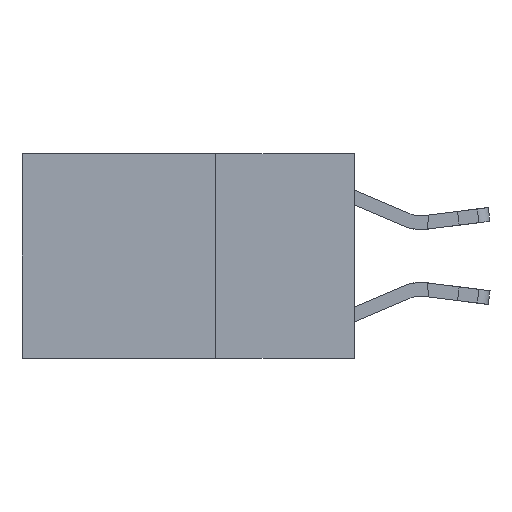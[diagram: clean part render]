
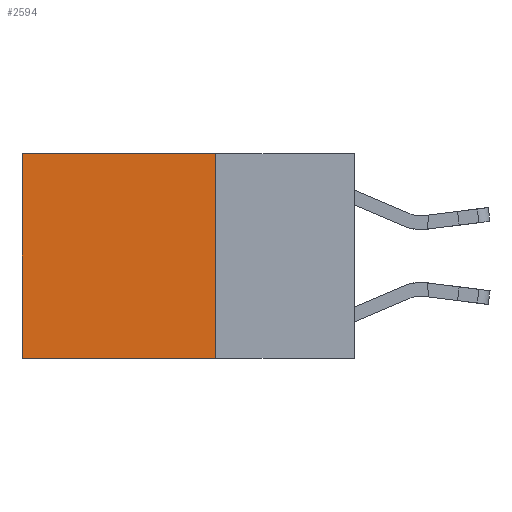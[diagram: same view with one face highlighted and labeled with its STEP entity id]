
A CAD part, left-side view. The second image highlights one B-rep face of the part: STEP entity #2594.
In plain terms, the highlighted planar face has unit normal (-1, 0, 0).
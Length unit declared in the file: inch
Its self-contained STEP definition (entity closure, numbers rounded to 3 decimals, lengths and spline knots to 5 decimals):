
#335 = ORIENTED_EDGE ( 'NONE', *, *, #14577, .F. ) ;
#1038 = FACE_OUTER_BOUND ( 'NONE', #13668, .T. ) ;
#1666 = PLANE ( 'NONE',  #3285 ) ;
#1735 = CARTESIAN_POINT ( 'NONE',  ( 0.2625, 0.25, 0. ) ) ;
#1909 = CARTESIAN_POINT ( 'NONE',  ( 0.2625, 0.6, 0. ) ) ;
#2092 = VERTEX_POINT ( 'NONE', #3716 ) ;
#2224 = EDGE_CURVE ( 'NONE', #2092, #17939, #18681, .T. ) ;
#2594 = ADVANCED_FACE ( 'NONE', ( #1038 ), #1666, .F. ) ;
#2650 = LINE ( 'NONE', #3391, #6215 ) ;
#3251 = DIRECTION ( 'NONE',  ( 0., 0., -1. ) ) ;
#3285 = AXIS2_PLACEMENT_3D ( 'NONE', #1735, #12367, #3251 ) ;
#3361 = CARTESIAN_POINT ( 'NONE',  ( 0.2625, 0.25, 0. ) ) ;
#3391 = CARTESIAN_POINT ( 'NONE',  ( 0.2625, 0.25, 0. ) ) ;
#3416 = DIRECTION ( 'NONE',  ( 0., 0., -1. ) ) ;
#3716 = CARTESIAN_POINT ( 'NONE',  ( 0.2625, 0.25, -0.37 ) ) ;
#4648 = ORIENTED_EDGE ( 'NONE', *, *, #13166, .T. ) ;
#6148 = LINE ( 'NONE', #1909, #14195 ) ;
#6215 = VECTOR ( 'NONE', #15488, 39.37008 ) ;
#7209 = CARTESIAN_POINT ( 'NONE',  ( 0.2625, 0.6, 0. ) ) ;
#7550 = DIRECTION ( 'NONE',  ( 0., 1., 0. ) ) ;
#7702 = VECTOR ( 'NONE', #17535, 39.37008 ) ;
#7861 = VERTEX_POINT ( 'NONE', #7209 ) ;
#7956 = CARTESIAN_POINT ( 'NONE',  ( 0.2625, 0.6, -0.37 ) ) ;
#9544 = EDGE_CURVE ( 'NONE', #7861, #17939, #6148, .T. ) ;
#10501 = ORIENTED_EDGE ( 'NONE', *, *, #9544, .T. ) ;
#11110 = ORIENTED_EDGE ( 'NONE', *, *, #2224, .F. ) ;
#12367 = DIRECTION ( 'NONE',  ( 1., 0., 0. ) ) ;
#12652 = VERTEX_POINT ( 'NONE', #3361 ) ;
#13166 = EDGE_CURVE ( 'NONE', #12652, #7861, #15707, .T. ) ;
#13668 = EDGE_LOOP ( 'NONE', ( #10501, #11110, #335, #4648 ) ) ;
#14195 = VECTOR ( 'NONE', #3416, 39.37008 ) ;
#14577 = EDGE_CURVE ( 'NONE', #12652, #2092, #2650, .T. ) ;
#15488 = DIRECTION ( 'NONE',  ( 0., 0., -1. ) ) ;
#15515 = CARTESIAN_POINT ( 'NONE',  ( 0.2625, 0.25, 0. ) ) ;
#15707 = LINE ( 'NONE', #15515, #19126 ) ;
#16070 = CARTESIAN_POINT ( 'NONE',  ( 0.2625, 0.25, -0.37 ) ) ;
#17535 = DIRECTION ( 'NONE',  ( 0., 1., 0. ) ) ;
#17939 = VERTEX_POINT ( 'NONE', #7956 ) ;
#18681 = LINE ( 'NONE', #16070, #7702 ) ;
#19126 = VECTOR ( 'NONE', #7550, 39.37008 ) ;
